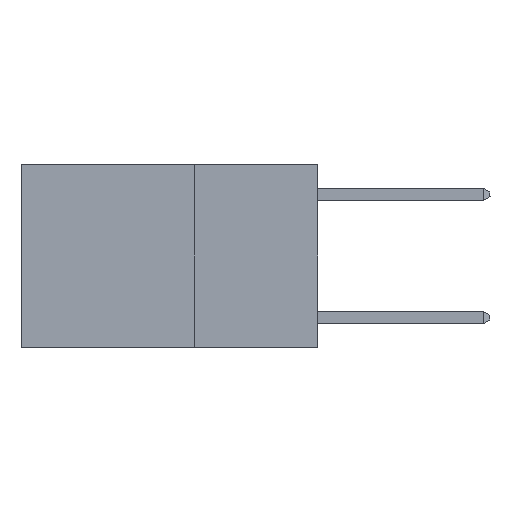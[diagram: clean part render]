
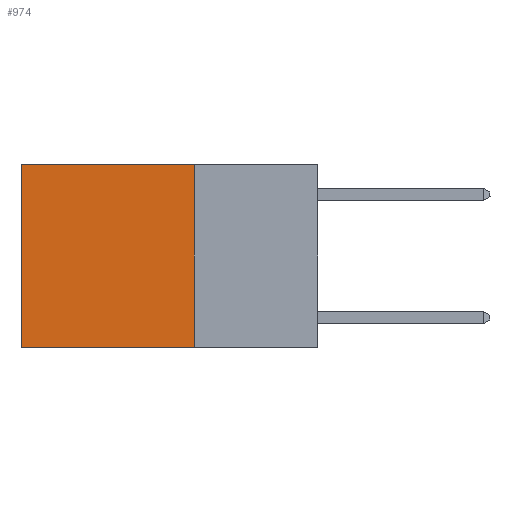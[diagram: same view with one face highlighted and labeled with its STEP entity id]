
A CAD part, left-side view. The second image highlights one B-rep face of the part: STEP entity #974.
In plain terms, the highlighted planar face has unit normal (-1, 0, 0).
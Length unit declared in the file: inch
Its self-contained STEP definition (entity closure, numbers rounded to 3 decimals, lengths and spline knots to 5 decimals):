
#974 = ADVANCED_FACE ( 'NONE', ( #17017 ), #12059, .F. ) ;
#1750 = VERTEX_POINT ( 'NONE', #10530 ) ;
#1841 = LINE ( 'NONE', #16153, #19744 ) ;
#2149 = VERTEX_POINT ( 'NONE', #14983 ) ;
#2245 = DIRECTION ( 'NONE',  ( 0., 0., -1. ) ) ;
#2510 = LINE ( 'NONE', #7007, #14653 ) ;
#2950 = CARTESIAN_POINT ( 'NONE',  ( 0.2625, 0.25, -0.37 ) ) ;
#3417 = CARTESIAN_POINT ( 'NONE',  ( 0.2625, 0.6, 0. ) ) ;
#4009 = DIRECTION ( 'NONE',  ( 0., 0., -1. ) ) ;
#4133 = EDGE_CURVE ( 'NONE', #16251, #2149, #8541, .T. ) ;
#4198 = CARTESIAN_POINT ( 'NONE',  ( 0.2625, 0.25, 0. ) ) ;
#6582 = DIRECTION ( 'NONE',  ( 0., 1., 0. ) ) ;
#7007 = CARTESIAN_POINT ( 'NONE',  ( 0.2625, 0.25, 0. ) ) ;
#8541 = LINE ( 'NONE', #3417, #9727 ) ;
#8685 = DIRECTION ( 'NONE',  ( 1., 0., 0. ) ) ;
#9214 = EDGE_CURVE ( 'NONE', #1750, #16721, #2510, .T. ) ;
#9540 = EDGE_CURVE ( 'NONE', #16721, #2149, #11216, .T. ) ;
#9727 = VECTOR ( 'NONE', #2245, 39.37008 ) ;
#10304 = VECTOR ( 'NONE', #6582, 39.37008 ) ;
#10530 = CARTESIAN_POINT ( 'NONE',  ( 0.2625, 0.25, 0. ) ) ;
#10610 = CARTESIAN_POINT ( 'NONE',  ( 0.2625, 0.6, 0. ) ) ;
#11216 = LINE ( 'NONE', #13005, #10304 ) ;
#11557 = EDGE_LOOP ( 'NONE', ( #14414, #16003, #16892, #11789 ) ) ;
#11789 = ORIENTED_EDGE ( 'NONE', *, *, #15405, .T. ) ;
#12059 = PLANE ( 'NONE',  #14545 ) ;
#12256 = DIRECTION ( 'NONE',  ( 0., 1., 0. ) ) ;
#13005 = CARTESIAN_POINT ( 'NONE',  ( 0.2625, 0.25, -0.37 ) ) ;
#14414 = ORIENTED_EDGE ( 'NONE', *, *, #4133, .T. ) ;
#14545 = AXIS2_PLACEMENT_3D ( 'NONE', #4198, #8685, #15268 ) ;
#14653 = VECTOR ( 'NONE', #4009, 39.37008 ) ;
#14983 = CARTESIAN_POINT ( 'NONE',  ( 0.2625, 0.6, -0.37 ) ) ;
#15268 = DIRECTION ( 'NONE',  ( 0., 0., -1. ) ) ;
#15405 = EDGE_CURVE ( 'NONE', #1750, #16251, #1841, .T. ) ;
#16003 = ORIENTED_EDGE ( 'NONE', *, *, #9540, .F. ) ;
#16153 = CARTESIAN_POINT ( 'NONE',  ( 0.2625, 0.25, 0. ) ) ;
#16251 = VERTEX_POINT ( 'NONE', #10610 ) ;
#16721 = VERTEX_POINT ( 'NONE', #2950 ) ;
#16892 = ORIENTED_EDGE ( 'NONE', *, *, #9214, .F. ) ;
#17017 = FACE_OUTER_BOUND ( 'NONE', #11557, .T. ) ;
#19744 = VECTOR ( 'NONE', #12256, 39.37008 ) ;
